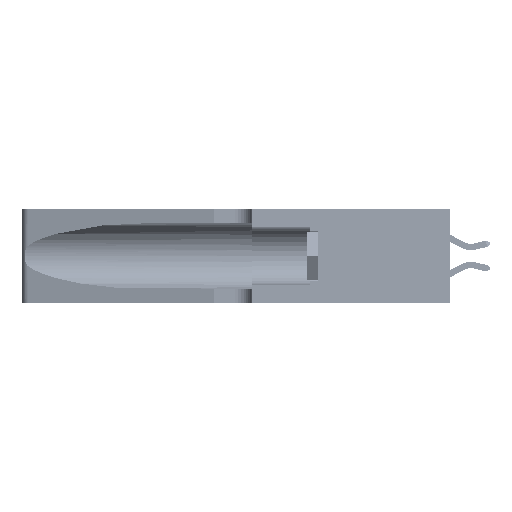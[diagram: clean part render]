
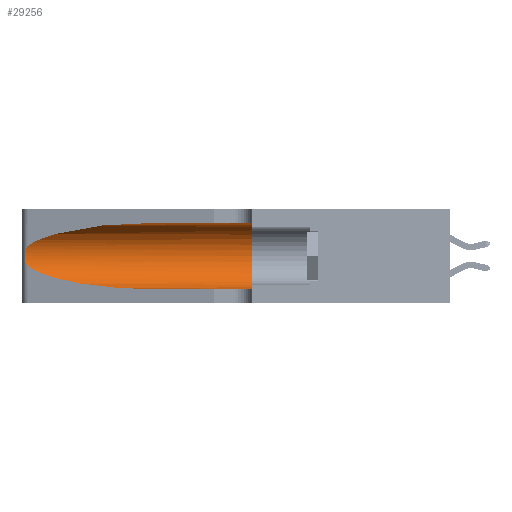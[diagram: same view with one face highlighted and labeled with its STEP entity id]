
A CAD part, left-side view. The second image highlights one B-rep face of the part: STEP entity #29256.
In plain terms, the highlighted cylindrical face has radius 3.308 mm (diameter 6.617 mm), a partial arc.
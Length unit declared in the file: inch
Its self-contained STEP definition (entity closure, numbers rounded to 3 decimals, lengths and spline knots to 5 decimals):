
#662 = CARTESIAN_POINT ( 'NONE',  ( 0.1305, 0.72297, 0.31525 ) ) ;
#1105 = VERTEX_POINT ( 'NONE', #28439 ) ;
#2931 = CARTESIAN_POINT ( 'NONE',  ( 0.25555, 1.22994, 0.2215 ) ) ;
#3088 = CARTESIAN_POINT ( 'NONE',  ( 0.25856, 1.23593, 0.16098 ) ) ;
#3279 = EDGE_CURVE ( 'NONE', #24791, #37963, #34841, .T. ) ;
#4749 = CARTESIAN_POINT ( 'NONE',  ( 0.18966, 0.96281, 0.05475 ) ) ;
#5610 = DIRECTION ( 'NONE',  ( 0., 1., 0. ) ) ;
#5717 = DIRECTION ( 'NONE',  ( 0., 0., -1. ) ) ;
#6663 = EDGE_CURVE ( 'NONE', #1105, #40588, #8679, .T. ) ;
#6877 = CARTESIAN_POINT ( 'NONE',  ( 0.25639, 1.23186, 0.15144 ) ) ;
#7551 = CARTESIAN_POINT ( 'NONE',  ( 0.2373, 1.15595, 0.28018 ) ) ;
#7617 = CARTESIAN_POINT ( 'NONE',  ( 0.1305, 0.72297, 0.05475 ) ) ;
#8679 = CIRCLE ( 'NONE', #32558, 0.13025 ) ;
#9840 = ORIENTED_EDGE ( 'NONE', *, *, #12365, .F. ) ;
#10253 =( BOUNDED_CURVE ( )  B_SPLINE_CURVE ( 3, ( #42019, #15940, #4749, #31051 ),
 .UNSPECIFIED., .F., .F. ) 
 B_SPLINE_CURVE_WITH_KNOTS ( ( 4, 4 ),
 ( 3.44316, 4.71239 ),
 .UNSPECIFIED. ) 
 CURVE ( )  GEOMETRIC_REPRESENTATION_ITEM ( )  RATIONAL_B_SPLINE_CURVE ( ( 1., 0.87, 0.87, 1. ) ) 
 REPRESENTATION_ITEM ( '' )  );
#10639 = CARTESIAN_POINT ( 'NONE',  ( 0.25487, 1.22718, 0.14631 ) ) ;
#10968 = AXIS2_PLACEMENT_3D ( 'NONE', #35709, #46887, #5717 ) ;
#11312 = CARTESIAN_POINT ( 'NONE',  ( 0.25487, 1.22718, 0.22369 ) ) ;
#12365 = EDGE_CURVE ( 'NONE', #24791, #1105, #29719, .T. ) ;
#13977 = ORIENTED_EDGE ( 'NONE', *, *, #3279, .T. ) ;
#14097 = CARTESIAN_POINT ( 'NONE',  ( 0.25487, 1.22718, 0.22369 ) ) ;
#14260 = CARTESIAN_POINT ( 'NONE',  ( 0.25639, 1.23184, 0.21858 ) ) ;
#14285 = EDGE_LOOP ( 'NONE', ( #13977, #30457, #20488, #43138, #29871, #9840 ) ) ;
#15940 = CARTESIAN_POINT ( 'NONE',  ( 0.2373, 1.15595, 0.08982 ) ) ;
#17073 = CARTESIAN_POINT ( 'NONE',  ( 0.1305, 1.61858, 0.05475 ) ) ;
#18059 = CARTESIAN_POINT ( 'NONE',  ( 0.25854, 1.2359, 0.20912 ) ) ;
#19025 = B_SPLINE_CURVE_WITH_KNOTS ( 'NONE', 3,
 ( #14097, #2931, #14260, #40388, #18059, #44087, #21881, #47839, #25662, #3088, #29433, #6877, #33111, #10639 ),
 .UNSPECIFIED., .F., .F.,
 ( 4, 2, 2, 2, 2, 2, 4 ),
 ( 0., 0.00027, 0.00053, 0.00107, 0.0016, 0.00187, 0.00214 ),
 .UNSPECIFIED. ) ;
#20022 = VECTOR ( 'NONE', #43116, 39.37008 ) ;
#20341 = CARTESIAN_POINT ( 'NONE',  ( 0.1305, 0.35, 0.05475 ) ) ;
#20488 = ORIENTED_EDGE ( 'NONE', *, *, #44155, .T. ) ;
#21881 = CARTESIAN_POINT ( 'NONE',  ( 0.26075, 1.23896, 0.19203 ) ) ;
#23726 = CARTESIAN_POINT ( 'NONE',  ( 0.25487, 1.22718, 0.22369 ) ) ;
#24428 = FACE_OUTER_BOUND ( 'NONE', #14285, .T. ) ;
#24791 = VERTEX_POINT ( 'NONE', #662 ) ;
#25662 = CARTESIAN_POINT ( 'NONE',  ( 0.26017, 1.23833, 0.17102 ) ) ;
#26256 = EDGE_CURVE ( 'NONE', #48345, #40588, #39827, .T. ) ;
#28179 = CARTESIAN_POINT ( 'NONE',  ( 0.1305, 0.35, 0.185 ) ) ;
#28439 = CARTESIAN_POINT ( 'NONE',  ( 0.1305, 0.35, 0.31525 ) ) ;
#28552 = VECTOR ( 'NONE', #45477, 39.37008 ) ;
#29256 = ADVANCED_FACE ( 'NONE', ( #24428 ), #42972, .F. ) ;
#29433 = CARTESIAN_POINT ( 'NONE',  ( 0.25789, 1.23486, 0.15765 ) ) ;
#29719 = LINE ( 'NONE', #41751, #28552 ) ;
#29871 = ORIENTED_EDGE ( 'NONE', *, *, #6663, .F. ) ;
#30457 = ORIENTED_EDGE ( 'NONE', *, *, #42046, .T. ) ;
#31051 = CARTESIAN_POINT ( 'NONE',  ( 0.1305, 0.72297, 0.05475 ) ) ;
#31916 = DIRECTION ( 'NONE',  ( 0., 0., 1. ) ) ;
#32558 = AXIS2_PLACEMENT_3D ( 'NONE', #28179, #5610, #31916 ) ;
#33111 = CARTESIAN_POINT ( 'NONE',  ( 0.25555, 1.22993, 0.14849 ) ) ;
#33762 = CARTESIAN_POINT ( 'NONE',  ( 0.18966, 0.96281, 0.31525 ) ) ;
#34841 =( BOUNDED_CURVE ( )  B_SPLINE_CURVE ( 3, ( #38735, #33762, #7551, #11312 ),
 .UNSPECIFIED., .F., .F. ) 
 B_SPLINE_CURVE_WITH_KNOTS ( ( 4, 4 ),
 ( 1.5708, 2.84003 ),
 .UNSPECIFIED. ) 
 CURVE ( )  GEOMETRIC_REPRESENTATION_ITEM ( )  RATIONAL_B_SPLINE_CURVE ( ( 1., 0.87, 0.87, 1. ) ) 
 REPRESENTATION_ITEM ( '' )  );
#35709 = CARTESIAN_POINT ( 'NONE',  ( 0.1305, 1.61858, 0.185 ) ) ;
#37963 = VERTEX_POINT ( 'NONE', #23726 ) ;
#38735 = CARTESIAN_POINT ( 'NONE',  ( 0.1305, 0.72297, 0.31525 ) ) ;
#39827 = LINE ( 'NONE', #17073, #20022 ) ;
#40388 = CARTESIAN_POINT ( 'NONE',  ( 0.25787, 1.23484, 0.2124 ) ) ;
#40556 = CARTESIAN_POINT ( 'NONE',  ( 0.25487, 1.22718, 0.14631 ) ) ;
#40588 = VERTEX_POINT ( 'NONE', #20341 ) ;
#41751 = CARTESIAN_POINT ( 'NONE',  ( 0.1305, 1.61858, 0.31525 ) ) ;
#42019 = CARTESIAN_POINT ( 'NONE',  ( 0.25487, 1.22718, 0.14631 ) ) ;
#42046 = EDGE_CURVE ( 'NONE', #37963, #47009, #19025, .T. ) ;
#42972 = CYLINDRICAL_SURFACE ( 'NONE', #10968, 0.13025 ) ;
#43116 = DIRECTION ( 'NONE',  ( 0., -1., 0. ) ) ;
#43138 = ORIENTED_EDGE ( 'NONE', *, *, #26256, .T. ) ;
#44087 = CARTESIAN_POINT ( 'NONE',  ( 0.26018, 1.23835, 0.19895 ) ) ;
#44155 = EDGE_CURVE ( 'NONE', #47009, #48345, #10253, .T. ) ;
#45477 = DIRECTION ( 'NONE',  ( 0., -1., 0. ) ) ;
#46887 = DIRECTION ( 'NONE',  ( 0., -1., 0. ) ) ;
#47009 = VERTEX_POINT ( 'NONE', #40556 ) ;
#47839 = CARTESIAN_POINT ( 'NONE',  ( 0.26075, 1.23896, 0.178 ) ) ;
#48345 = VERTEX_POINT ( 'NONE', #7617 ) ;
